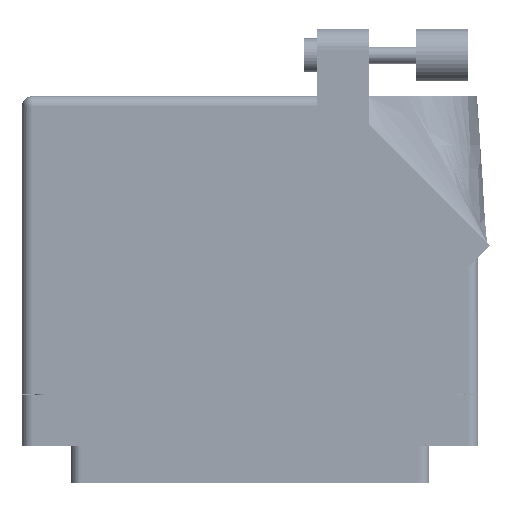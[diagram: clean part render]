
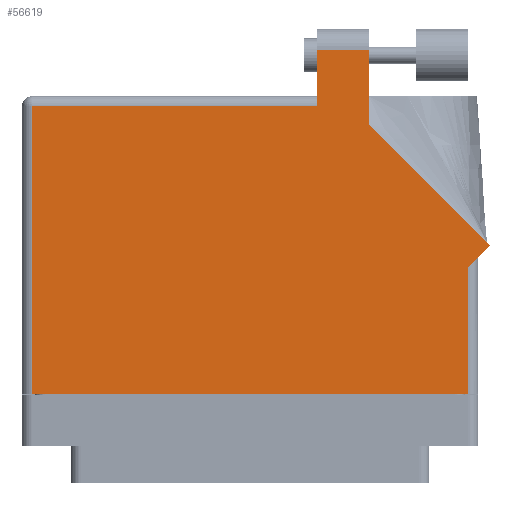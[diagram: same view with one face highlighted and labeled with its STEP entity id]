
A CAD part, front view. The second image highlights one B-rep face of the part: STEP entity #56619.
In plain terms, the highlighted face is planar.
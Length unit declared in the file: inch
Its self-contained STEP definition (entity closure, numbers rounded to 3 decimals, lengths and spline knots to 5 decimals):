
#193 = LINE ( 'NONE', #27846, #54540 ) ;
#869 = VERTEX_POINT ( 'NONE', #37675 ) ;
#1801 = CARTESIAN_POINT ( 'NONE',  ( 1.297, -0.1, 0.617 ) ) ;
#2353 = ORIENTED_EDGE ( 'NONE', *, *, #59674, .T. ) ;
#2463 = ORIENTED_EDGE ( 'NONE', *, *, #54462, .T. ) ;
#2717 = EDGE_CURVE ( 'NONE', #63788, #62302, #37997, .T. ) ;
#3614 = DIRECTION ( 'NONE',  ( 0., 1., 0. ) ) ;
#4975 = DIRECTION ( 'NONE',  ( -1., 0., 0. ) ) ;
#5754 = VERTEX_POINT ( 'NONE', #5900 ) ;
#5900 = CARTESIAN_POINT ( 'NONE',  ( 1.297, 0.653, 0.617 ) ) ;
#6333 = EDGE_CURVE ( 'NONE', #5754, #46756, #193, .T. ) ;
#8010 = CARTESIAN_POINT ( 'NONE',  ( -1.297, -0.1, 0.617 ) ) ;
#8887 = VECTOR ( 'NONE', #44961, 39.37008 ) ;
#9191 = VECTOR ( 'NONE', #59161, 39.37008 ) ;
#10203 = CARTESIAN_POINT ( 'NONE',  ( -1.359, -0.1, 0.617 ) ) ;
#10691 = DIRECTION ( 'NONE',  ( -1., 0., 0. ) ) ;
#10786 = VERTEX_POINT ( 'NONE', #1801 ) ;
#12370 = CARTESIAN_POINT ( 'NONE',  ( 0.706, 1.50942, 0.617 ) ) ;
#13184 = ORIENTED_EDGE ( 'NONE', *, *, #66543, .T. ) ;
#14083 = LINE ( 'NONE', #30498, #53957 ) ;
#17454 = PLANE ( 'NONE',  #59429 ) ;
#18005 = DIRECTION ( 'NONE',  ( 1., 0., 0. ) ) ;
#18117 = LINE ( 'NONE', #46608, #56345 ) ;
#18204 = EDGE_LOOP ( 'NONE', ( #52345, #47357, #55324, #13184, #45624, #2463, #2353, #32250, #27429 ) ) ;
#19032 = LINE ( 'NONE', #8010, #28309 ) ;
#24659 = VERTEX_POINT ( 'NONE', #53313 ) ;
#25147 = FACE_OUTER_BOUND ( 'NONE', #18204, .T. ) ;
#25386 = VECTOR ( 'NONE', #3614, 39.37008 ) ;
#25741 = VECTOR ( 'NONE', #4975, 39.37008 ) ;
#27429 = ORIENTED_EDGE ( 'NONE', *, *, #58110, .T. ) ;
#27440 = CARTESIAN_POINT ( 'NONE',  ( 1.42971, 0.78571, 0.617 ) ) ;
#27846 = CARTESIAN_POINT ( 'NONE',  ( 1.359, 0.715, 0.617 ) ) ;
#28309 = VECTOR ( 'NONE', #45891, 39.37008 ) ;
#28313 = DIRECTION ( 'NONE',  ( 0.707, 0.707, 0. ) ) ;
#28807 = EDGE_CURVE ( 'NONE', #24659, #50470, #35220, .T. ) ;
#29013 = EDGE_CURVE ( 'NONE', #64809, #869, #19032, .T. ) ;
#30498 = CARTESIAN_POINT ( 'NONE',  ( 0.399, 1.95, 0.617 ) ) ;
#31344 = CARTESIAN_POINT ( 'NONE',  ( 0.399, 1.613, 0.617 ) ) ;
#32250 = ORIENTED_EDGE ( 'NONE', *, *, #6333, .T. ) ;
#32956 = CARTESIAN_POINT ( 'NONE',  ( 0.706, 1.95, 0.617 ) ) ;
#33824 = DIRECTION ( 'NONE',  ( 0., 0., -1. ) ) ;
#35220 = LINE ( 'NONE', #50453, #8887 ) ;
#37675 = CARTESIAN_POINT ( 'NONE',  ( -1.297, -0.1, 0.617 ) ) ;
#37997 = LINE ( 'NONE', #69628, #9191 ) ;
#44233 = DIRECTION ( 'NONE',  ( -1., 0., 0. ) ) ;
#44961 = DIRECTION ( 'NONE',  ( 0., -1., 0. ) ) ;
#45624 = ORIENTED_EDGE ( 'NONE', *, *, #29013, .T. ) ;
#45891 = DIRECTION ( 'NONE',  ( 0., -1., 0. ) ) ;
#46536 = VECTOR ( 'NONE', #18005, 39.37008 ) ;
#46608 = CARTESIAN_POINT ( 'NONE',  ( 1.42971, 0.78571, 0.617 ) ) ;
#46756 = VERTEX_POINT ( 'NONE', #27440 ) ;
#47357 = ORIENTED_EDGE ( 'NONE', *, *, #64845, .T. ) ;
#48552 = CARTESIAN_POINT ( 'NONE',  ( -1.359, 1.613, 0.617 ) ) ;
#50453 = CARTESIAN_POINT ( 'NONE',  ( 0.399, 1.675, 0.617 ) ) ;
#50470 = VERTEX_POINT ( 'NONE', #31344 ) ;
#52345 = ORIENTED_EDGE ( 'NONE', *, *, #2717, .T. ) ;
#52600 = LINE ( 'NONE', #57240, #25386 ) ;
#53313 = CARTESIAN_POINT ( 'NONE',  ( 0.399, 1.95, 0.617 ) ) ;
#53957 = VECTOR ( 'NONE', #10691, 39.37008 ) ;
#54462 = EDGE_CURVE ( 'NONE', #869, #10786, #64465, .T. ) ;
#54540 = VECTOR ( 'NONE', #28313, 39.37008 ) ;
#55324 = ORIENTED_EDGE ( 'NONE', *, *, #28807, .T. ) ;
#55475 = CARTESIAN_POINT ( 'NONE',  ( -1.359, 1.675, 0.617 ) ) ;
#56345 = VECTOR ( 'NONE', #62790, 39.37008 ) ;
#56619 = ADVANCED_FACE ( 'NONE', ( #25147 ), #17454, .F. ) ;
#57240 = CARTESIAN_POINT ( 'NONE',  ( 1.297, 0.715, 0.617 ) ) ;
#57360 = CARTESIAN_POINT ( 'NONE',  ( -1.297, 1.613, 0.617 ) ) ;
#58110 = EDGE_CURVE ( 'NONE', #46756, #63788, #18117, .T. ) ;
#59161 = DIRECTION ( 'NONE',  ( 0., 1., 0. ) ) ;
#59429 = AXIS2_PLACEMENT_3D ( 'NONE', #55475, #33824, #44233 ) ;
#59674 = EDGE_CURVE ( 'NONE', #10786, #5754, #52600, .T. ) ;
#62302 = VERTEX_POINT ( 'NONE', #32956 ) ;
#62790 = DIRECTION ( 'NONE',  ( -0.707, 0.707, 0. ) ) ;
#63788 = VERTEX_POINT ( 'NONE', #12370 ) ;
#64465 = LINE ( 'NONE', #10203, #46536 ) ;
#64809 = VERTEX_POINT ( 'NONE', #57360 ) ;
#64845 = EDGE_CURVE ( 'NONE', #62302, #24659, #14083, .T. ) ;
#65672 = LINE ( 'NONE', #48552, #25741 ) ;
#66543 = EDGE_CURVE ( 'NONE', #50470, #64809, #65672, .T. ) ;
#69628 = CARTESIAN_POINT ( 'NONE',  ( 0.706, 1.50942, 0.617 ) ) ;
